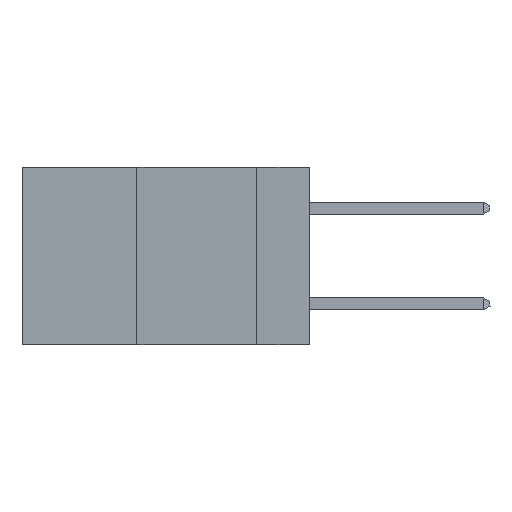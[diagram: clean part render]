
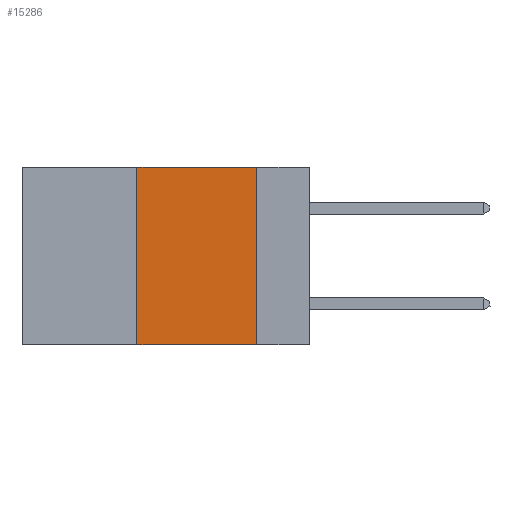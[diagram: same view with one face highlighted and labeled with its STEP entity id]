
A CAD part, left-side view. The second image highlights one B-rep face of the part: STEP entity #15286.
In plain terms, the highlighted planar face has unit normal (-1, 0, 0).
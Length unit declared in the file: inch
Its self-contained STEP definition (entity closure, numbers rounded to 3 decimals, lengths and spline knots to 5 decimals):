
#6 = EDGE_CURVE ( 'NONE', #14664, #10954, #14093, .T. ) ;
#505 = DIRECTION ( 'NONE',  ( 0., 0., 1. ) ) ;
#1479 = LINE ( 'NONE', #7596, #15661 ) ;
#2676 = CARTESIAN_POINT ( 'NONE',  ( 0., 0.6, 0. ) ) ;
#2859 = CARTESIAN_POINT ( 'NONE',  ( 0., 0.36, 0. ) ) ;
#3000 = CARTESIAN_POINT ( 'NONE',  ( 0., 0.36, 0. ) ) ;
#3688 = AXIS2_PLACEMENT_3D ( 'NONE', #2676, #9587, #8449 ) ;
#4253 = CARTESIAN_POINT ( 'NONE',  ( 0., 0.6, -0.37 ) ) ;
#5605 = DIRECTION ( 'NONE',  ( 0., -1., 0. ) ) ;
#5943 = CARTESIAN_POINT ( 'NONE',  ( 0., 0.11, -0.37 ) ) ;
#6477 = ORIENTED_EDGE ( 'NONE', *, *, #8002, .F. ) ;
#7596 = CARTESIAN_POINT ( 'NONE',  ( 0., 0.11, 0. ) ) ;
#8002 = EDGE_CURVE ( 'NONE', #10954, #12308, #1479, .T. ) ;
#8106 = PLANE ( 'NONE',  #3688 ) ;
#8449 = DIRECTION ( 'NONE',  ( 0., 0., -1. ) ) ;
#9040 = DIRECTION ( 'NONE',  ( 0., -1., 0. ) ) ;
#9587 = DIRECTION ( 'NONE',  ( 1., 0., 0. ) ) ;
#9930 = EDGE_CURVE ( 'NONE', #14152, #14664, #17031, .T. ) ;
#10488 = VECTOR ( 'NONE', #9040, 39.37008 ) ;
#10750 = ORIENTED_EDGE ( 'NONE', *, *, #13406, .T. ) ;
#10752 = LINE ( 'NONE', #4253, #15439 ) ;
#10954 = VERTEX_POINT ( 'NONE', #11493 ) ;
#11493 = CARTESIAN_POINT ( 'NONE',  ( 0., 0.11, 0. ) ) ;
#11673 = DIRECTION ( 'NONE',  ( 0., 0., -1. ) ) ;
#12138 = ORIENTED_EDGE ( 'NONE', *, *, #9930, .F. ) ;
#12308 = VERTEX_POINT ( 'NONE', #5943 ) ;
#12463 = CARTESIAN_POINT ( 'NONE',  ( 0., 0.36, -0.37 ) ) ;
#12544 = VECTOR ( 'NONE', #505, 39.37008 ) ;
#12563 = FACE_OUTER_BOUND ( 'NONE', #16134, .T. ) ;
#13406 = EDGE_CURVE ( 'NONE', #14152, #12308, #10752, .T. ) ;
#14093 = LINE ( 'NONE', #14371, #10488 ) ;
#14152 = VERTEX_POINT ( 'NONE', #12463 ) ;
#14371 = CARTESIAN_POINT ( 'NONE',  ( 0., 0.6, 0. ) ) ;
#14664 = VERTEX_POINT ( 'NONE', #2859 ) ;
#15242 = ORIENTED_EDGE ( 'NONE', *, *, #6, .F. ) ;
#15286 = ADVANCED_FACE ( 'NONE', ( #12563 ), #8106, .F. ) ;
#15439 = VECTOR ( 'NONE', #5605, 39.37008 ) ;
#15661 = VECTOR ( 'NONE', #11673, 39.37008 ) ;
#16134 = EDGE_LOOP ( 'NONE', ( #6477, #15242, #12138, #10750 ) ) ;
#17031 = LINE ( 'NONE', #3000, #12544 ) ;
